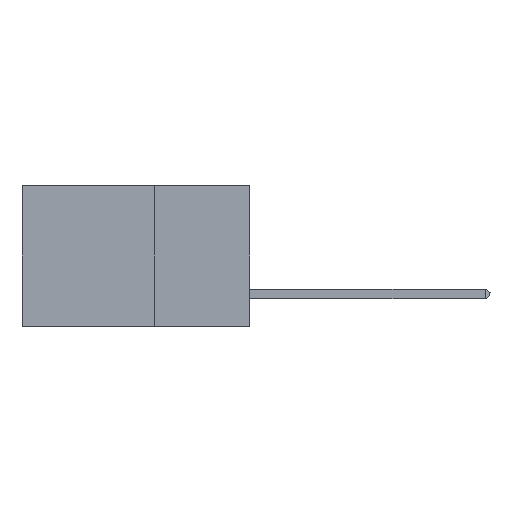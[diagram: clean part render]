
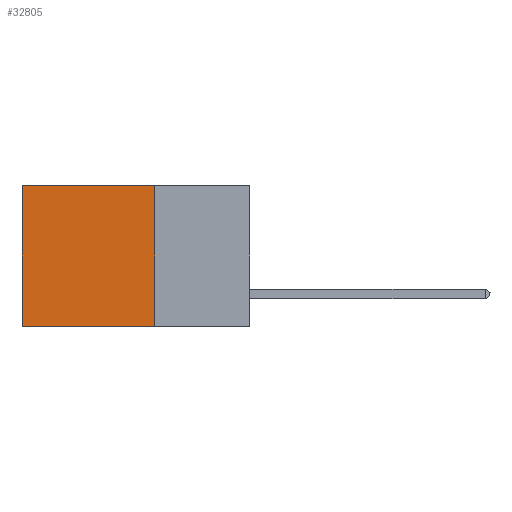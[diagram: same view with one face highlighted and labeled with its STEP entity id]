
A CAD part, left-side view. The second image highlights one B-rep face of the part: STEP entity #32805.
In plain terms, the highlighted planar face has unit normal (-1, 0, 0).
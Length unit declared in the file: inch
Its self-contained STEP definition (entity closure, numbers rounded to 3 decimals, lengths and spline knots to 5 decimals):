
#251 = VERTEX_POINT ( 'NONE', #17838 ) ;
#1857 = LINE ( 'NONE', #11160, #39921 ) ;
#2290 = ORIENTED_EDGE ( 'NONE', *, *, #43350, .F. ) ;
#2813 = EDGE_CURVE ( 'NONE', #251, #10149, #46216, .T. ) ;
#4804 = EDGE_CURVE ( 'NONE', #251, #31809, #1857, .T. ) ;
#6852 = PLANE ( 'NONE',  #48802 ) ;
#10149 = VERTEX_POINT ( 'NONE', #13479 ) ;
#10399 = DIRECTION ( 'NONE',  ( 0., 0., -1. ) ) ;
#11160 = CARTESIAN_POINT ( 'NONE',  ( 0.2875, 0.25, 0. ) ) ;
#12472 = DIRECTION ( 'NONE',  ( 0., 1., 0. ) ) ;
#13363 = CARTESIAN_POINT ( 'NONE',  ( 0.2875, 0.6, -0.37 ) ) ;
#13479 = CARTESIAN_POINT ( 'NONE',  ( 0.2875, 0.6, 0. ) ) ;
#14373 = ORIENTED_EDGE ( 'NONE', *, *, #46903, .T. ) ;
#16599 = VECTOR ( 'NONE', #42890, 39.37008 ) ;
#17838 = CARTESIAN_POINT ( 'NONE',  ( 0.2875, 0.25, 0. ) ) ;
#18548 = VECTOR ( 'NONE', #12472, 39.37008 ) ;
#18751 = EDGE_LOOP ( 'NONE', ( #14373, #2290, #48131, #38929 ) ) ;
#21888 = DIRECTION ( 'NONE',  ( 1., 0., 0. ) ) ;
#25166 = LINE ( 'NONE', #47810, #18548 ) ;
#29815 = CARTESIAN_POINT ( 'NONE',  ( 0.2875, 0.25, 0. ) ) ;
#31571 = CARTESIAN_POINT ( 'NONE',  ( 0.2875, 0.25, 0. ) ) ;
#31809 = VERTEX_POINT ( 'NONE', #35479 ) ;
#32805 = ADVANCED_FACE ( 'NONE', ( #44175 ), #6852, .F. ) ;
#33907 = DIRECTION ( 'NONE',  ( 0., 0., -1. ) ) ;
#35479 = CARTESIAN_POINT ( 'NONE',  ( 0.2875, 0.25, -0.37 ) ) ;
#35661 = VECTOR ( 'NONE', #33907, 39.37008 ) ;
#38929 = ORIENTED_EDGE ( 'NONE', *, *, #2813, .T. ) ;
#39921 = VECTOR ( 'NONE', #50050, 39.37008 ) ;
#42890 = DIRECTION ( 'NONE',  ( 0., 1., 0. ) ) ;
#43350 = EDGE_CURVE ( 'NONE', #31809, #44397, #25166, .T. ) ;
#44175 = FACE_OUTER_BOUND ( 'NONE', #18751, .T. ) ;
#44397 = VERTEX_POINT ( 'NONE', #13363 ) ;
#46216 = LINE ( 'NONE', #31571, #16599 ) ;
#46903 = EDGE_CURVE ( 'NONE', #10149, #44397, #47162, .T. ) ;
#47162 = LINE ( 'NONE', #49309, #35661 ) ;
#47810 = CARTESIAN_POINT ( 'NONE',  ( 0.2875, 0.25, -0.37 ) ) ;
#48131 = ORIENTED_EDGE ( 'NONE', *, *, #4804, .F. ) ;
#48802 = AXIS2_PLACEMENT_3D ( 'NONE', #29815, #21888, #10399 ) ;
#49309 = CARTESIAN_POINT ( 'NONE',  ( 0.2875, 0.6, 0. ) ) ;
#50050 = DIRECTION ( 'NONE',  ( 0., 0., -1. ) ) ;
